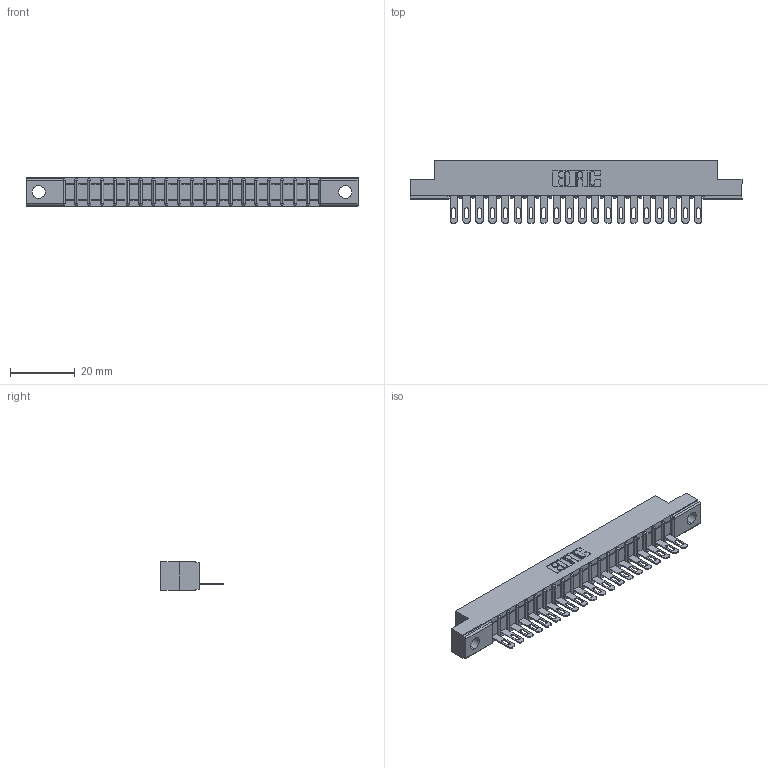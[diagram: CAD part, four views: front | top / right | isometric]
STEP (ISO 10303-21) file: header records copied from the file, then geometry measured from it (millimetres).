
FILE_DESCRIPTION (( 'STEP AP203' ), '1' );
FILE_NAME ('307-020-405-102.STEP', '2020-09-27T01:26:41', ( '' ), ( '' ), 'SwSTEP 2.0', 'SolidWorks 2020', '' );
FILE_SCHEMA (( 'CONFIG_CONTROL_DESIGN' ));
Length unit declared in the file: inch
Products named in the file (3): 307-020-405-102; 307 Part_.128 Dia Mounting Holes; 307-290-001_505
Assembly tree (21 placements, depth 2):
  307-020-405-102
    307 Part_.128 Dia Mounting Holes
    307-290-001_505  x20
Bounding box: 102.26 x 19.18 x 8.71 mm (x, y, z)
Volume: 6400.6 mm3; surface area: 9842.2 mm2
Topology: 21 solids, 21 shells, 1259 faces, 3563 edges, 2290 vertices
Faces by surface type: plane 790, cylinder 427, sphere 42
Entity records: 19834 total; most frequent: CARTESIAN_POINT 3332, ORIENTED_EDGE 3318, DIRECTION 3255, EDGE_CURVE 1659, LINE 1261, VECTOR 1261, VERTEX_POINT 1074, AXIS2_PLACEMENT_3D 997
